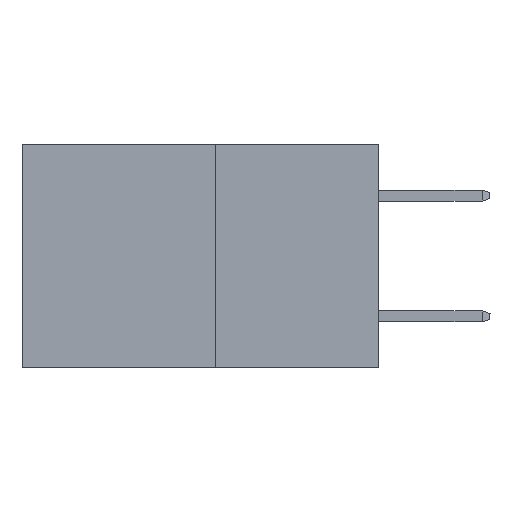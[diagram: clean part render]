
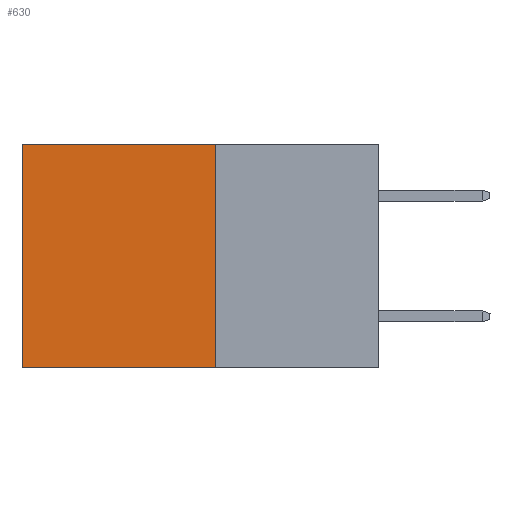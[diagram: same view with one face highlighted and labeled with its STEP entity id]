
A CAD part, left-side view. The second image highlights one B-rep face of the part: STEP entity #630.
In plain terms, the highlighted planar face has unit normal (-1, 0, 0).
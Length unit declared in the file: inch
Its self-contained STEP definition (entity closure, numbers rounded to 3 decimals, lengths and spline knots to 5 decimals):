
#247 = LINE ( 'NONE', #910, #3683 ) ;
#394 = CARTESIAN_POINT ( 'NONE',  ( 0.277, 0.59, -0.37 ) ) ;
#434 = CARTESIAN_POINT ( 'NONE',  ( 0.277, 0.59, -0.37 ) ) ;
#491 = AXIS2_PLACEMENT_3D ( 'NONE', #2387, #2486, #6093 ) ;
#630 = ADVANCED_FACE ( 'NONE', ( #8948 ), #5873, .F. ) ;
#910 = CARTESIAN_POINT ( 'NONE',  ( 0.277, 0.27, 0. ) ) ;
#914 = VERTEX_POINT ( 'NONE', #434 ) ;
#1839 = VERTEX_POINT ( 'NONE', #5153 ) ;
#2324 = VECTOR ( 'NONE', #6235, 39.37008 ) ;
#2387 = CARTESIAN_POINT ( 'NONE',  ( 0.277, 0.27, -0.37 ) ) ;
#2486 = DIRECTION ( 'NONE',  ( 1., 0., 0. ) ) ;
#2505 = VERTEX_POINT ( 'NONE', #3566 ) ;
#2539 = LINE ( 'NONE', #394, #2324 ) ;
#2695 = CARTESIAN_POINT ( 'NONE',  ( 0.277, 0.27, -0.37 ) ) ;
#3523 = DIRECTION ( 'NONE',  ( 0., 1., 0. ) ) ;
#3566 = CARTESIAN_POINT ( 'NONE',  ( 0.277, 0.27, -0.37 ) ) ;
#3683 = VECTOR ( 'NONE', #3523, 39.37008 ) ;
#3862 = DIRECTION ( 'NONE',  ( 0., 1., 0. ) ) ;
#3966 = EDGE_LOOP ( 'NONE', ( #4846, #9123, #4636, #5820 ) ) ;
#4244 = VECTOR ( 'NONE', #3862, 39.37008 ) ;
#4580 = LINE ( 'NONE', #9154, #6411 ) ;
#4636 = ORIENTED_EDGE ( 'NONE', *, *, #7653, .F. ) ;
#4716 = EDGE_CURVE ( 'NONE', #1839, #914, #2539, .T. ) ;
#4846 = ORIENTED_EDGE ( 'NONE', *, *, #4716, .T. ) ;
#5107 = CARTESIAN_POINT ( 'NONE',  ( 0.277, 0.27, 0. ) ) ;
#5153 = CARTESIAN_POINT ( 'NONE',  ( 0.277, 0.59, 0. ) ) ;
#5820 = ORIENTED_EDGE ( 'NONE', *, *, #7418, .T. ) ;
#5873 = PLANE ( 'NONE',  #491 ) ;
#6093 = DIRECTION ( 'NONE',  ( 0., 0., -1. ) ) ;
#6235 = DIRECTION ( 'NONE',  ( 0., 0., -1. ) ) ;
#6303 = LINE ( 'NONE', #2695, #4244 ) ;
#6411 = VECTOR ( 'NONE', #7632, 39.37008 ) ;
#6520 = VERTEX_POINT ( 'NONE', #5107 ) ;
#7007 = EDGE_CURVE ( 'NONE', #2505, #914, #6303, .T. ) ;
#7418 = EDGE_CURVE ( 'NONE', #6520, #1839, #247, .T. ) ;
#7632 = DIRECTION ( 'NONE',  ( 0., 0., -1. ) ) ;
#7653 = EDGE_CURVE ( 'NONE', #6520, #2505, #4580, .T. ) ;
#8948 = FACE_OUTER_BOUND ( 'NONE', #3966, .T. ) ;
#9123 = ORIENTED_EDGE ( 'NONE', *, *, #7007, .F. ) ;
#9154 = CARTESIAN_POINT ( 'NONE',  ( 0.277, 0.27, -0.37 ) ) ;
